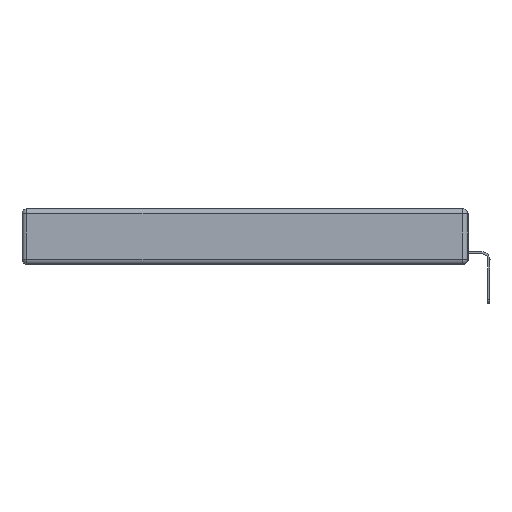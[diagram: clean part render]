
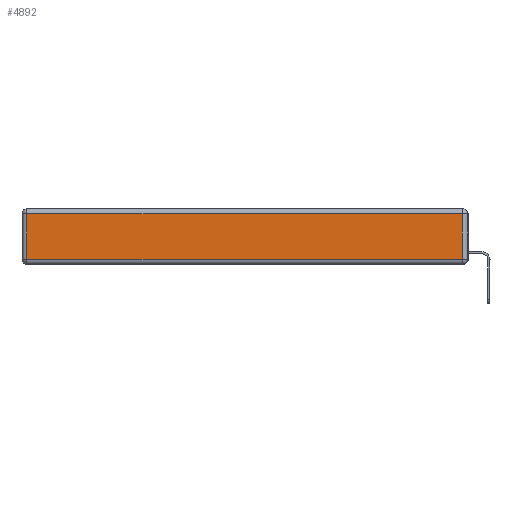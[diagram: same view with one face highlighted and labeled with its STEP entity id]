
A CAD part, left-side view. The second image highlights one B-rep face of the part: STEP entity #4892.
In plain terms, the highlighted planar face has unit normal (-1, 0, 0).
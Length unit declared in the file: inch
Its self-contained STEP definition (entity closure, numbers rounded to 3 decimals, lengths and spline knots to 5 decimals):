
#83 = LINE ( 'NONE', #1341, #4883 ) ;
#345 = VECTOR ( 'NONE', #5814, 39.37008 ) ;
#346 = CARTESIAN_POINT ( 'NONE',  ( 0., 2.75, -0.03 ) ) ;
#512 = CARTESIAN_POINT ( 'NONE',  ( 0., 2.72, -0.313 ) ) ;
#1103 = ORIENTED_EDGE ( 'NONE', *, *, #6821, .T. ) ;
#1217 = VERTEX_POINT ( 'NONE', #9233 ) ;
#1341 = CARTESIAN_POINT ( 'NONE',  ( 0., 0., -0.313 ) ) ;
#1487 = DIRECTION ( 'NONE',  ( 0., 0., -1. ) ) ;
#1701 = CARTESIAN_POINT ( 'NONE',  ( 0., 0.03, -0.03 ) ) ;
#2158 = VECTOR ( 'NONE', #5251, 39.37008 ) ;
#3083 = EDGE_CURVE ( 'NONE', #10953, #7172, #10182, .T. ) ;
#3405 = CARTESIAN_POINT ( 'NONE',  ( 0., 2.72, -0.343 ) ) ;
#4724 = DIRECTION ( 'NONE',  ( -1., 0., 0. ) ) ;
#4883 = VECTOR ( 'NONE', #10023, 39.37008 ) ;
#4892 = ADVANCED_FACE ( 'NONE', ( #9117 ), #6352, .T. ) ;
#4952 = CARTESIAN_POINT ( 'NONE',  ( 0., 2.72, -0.03 ) ) ;
#5251 = DIRECTION ( 'NONE',  ( 0., 1., 0. ) ) ;
#5548 = ORIENTED_EDGE ( 'NONE', *, *, #7171, .T. ) ;
#5791 = DIRECTION ( 'NONE',  ( 0., 0., 1. ) ) ;
#5814 = DIRECTION ( 'NONE',  ( 0., 0., 1. ) ) ;
#5949 = AXIS2_PLACEMENT_3D ( 'NONE', #7324, #4724, #5791 ) ;
#6012 = ORIENTED_EDGE ( 'NONE', *, *, #7634, .T. ) ;
#6332 = VERTEX_POINT ( 'NONE', #1701 ) ;
#6352 = PLANE ( 'NONE',  #5949 ) ;
#6622 = EDGE_LOOP ( 'NONE', ( #5548, #6012, #1103, #10850 ) ) ;
#6821 = EDGE_CURVE ( 'NONE', #6332, #10953, #9565, .T. ) ;
#6994 = VECTOR ( 'NONE', #1487, 39.37008 ) ;
#7171 = EDGE_CURVE ( 'NONE', #7172, #1217, #83, .T. ) ;
#7172 = VERTEX_POINT ( 'NONE', #512 ) ;
#7266 = LINE ( 'NONE', #8707, #345 ) ;
#7324 = CARTESIAN_POINT ( 'NONE',  ( 0., 0., -0.343 ) ) ;
#7634 = EDGE_CURVE ( 'NONE', #1217, #6332, #7266, .T. ) ;
#8707 = CARTESIAN_POINT ( 'NONE',  ( 0., 0.03, -0.343 ) ) ;
#9117 = FACE_OUTER_BOUND ( 'NONE', #6622, .T. ) ;
#9233 = CARTESIAN_POINT ( 'NONE',  ( 0., 0.03, -0.313 ) ) ;
#9565 = LINE ( 'NONE', #346, #2158 ) ;
#10023 = DIRECTION ( 'NONE',  ( 0., -1., 0. ) ) ;
#10182 = LINE ( 'NONE', #3405, #6994 ) ;
#10850 = ORIENTED_EDGE ( 'NONE', *, *, #3083, .T. ) ;
#10953 = VERTEX_POINT ( 'NONE', #4952 ) ;
